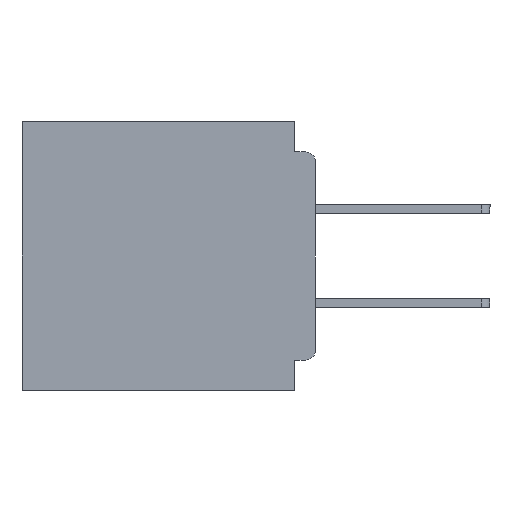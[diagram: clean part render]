
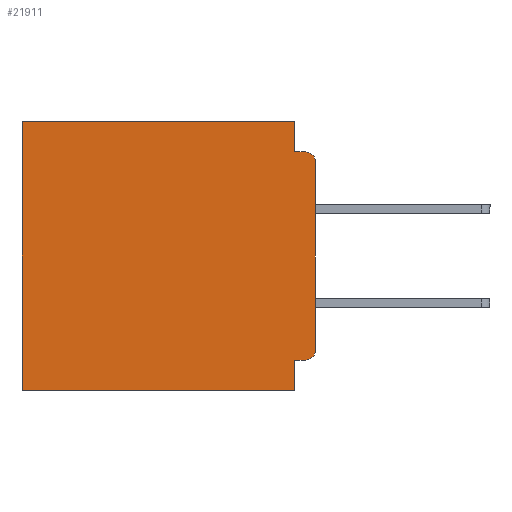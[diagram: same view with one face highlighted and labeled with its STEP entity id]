
A CAD part, left-side view. The second image highlights one B-rep face of the part: STEP entity #21911.
In plain terms, the highlighted planar face has unit normal (-1, 0, 0).
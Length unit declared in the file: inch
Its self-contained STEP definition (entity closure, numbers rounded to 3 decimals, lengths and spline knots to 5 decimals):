
#25 = EDGE_CURVE ( 'NONE', #33860, #26058, #36874, .T. ) ;
#89 = VERTEX_POINT ( 'NONE', #27693 ) ;
#97 = CARTESIAN_POINT ( 'NONE',  ( 0.3, 0.015, -0.06 ) ) ;
#1102 = VECTOR ( 'NONE', #43353, 39.37008 ) ;
#1605 = EDGE_CURVE ( 'NONE', #33860, #23498, #42872, .T. ) ;
#1631 = DIRECTION ( 'NONE',  ( 0., 0., -1. ) ) ;
#1905 = EDGE_CURVE ( 'NONE', #11350, #89, #7757, .T. ) ;
#2733 = ORIENTED_EDGE ( 'NONE', *, *, #29844, .F. ) ;
#2959 = DIRECTION ( 'NONE',  ( -1., 0., 0. ) ) ;
#3622 = CARTESIAN_POINT ( 'NONE',  ( 0.3, 0., -0.34 ) ) ;
#4730 = VECTOR ( 'NONE', #41948, 39.37008 ) ;
#5272 = CARTESIAN_POINT ( 'NONE',  ( 0.3, 0., -0.06 ) ) ;
#5467 = CARTESIAN_POINT ( 'NONE',  ( 0.3, 0.031, 0. ) ) ;
#6427 = AXIS2_PLACEMENT_3D ( 'NONE', #97, #45173, #18977 ) ;
#6617 = CARTESIAN_POINT ( 'NONE',  ( 0.3, 0.031, -0.4 ) ) ;
#6880 = ORIENTED_EDGE ( 'NONE', *, *, #1605, .F. ) ;
#7757 = LINE ( 'NONE', #12487, #46294 ) ;
#8088 = DIRECTION ( 'NONE',  ( 0., -1., 0. ) ) ;
#8098 = CARTESIAN_POINT ( 'NONE',  ( 0.3, 0.437, -0.4 ) ) ;
#9682 = CIRCLE ( 'NONE', #31097, 0.015 ) ;
#10049 = VERTEX_POINT ( 'NONE', #12297 ) ;
#11350 = VERTEX_POINT ( 'NONE', #5467 ) ;
#11752 = EDGE_LOOP ( 'NONE', ( #6880, #23285, #32112, #19750, #48287, #26219, #25047, #2733, #31502, #19133 ) ) ;
#11902 = VECTOR ( 'NONE', #24379, 39.37008 ) ;
#12297 = CARTESIAN_POINT ( 'NONE',  ( 0.3, 0.031, -0.045 ) ) ;
#12487 = CARTESIAN_POINT ( 'NONE',  ( 0.3, 0., 0. ) ) ;
#13491 = CARTESIAN_POINT ( 'NONE',  ( 0.3, 0.031, 0. ) ) ;
#15126 = EDGE_CURVE ( 'NONE', #20086, #39308, #40803, .T. ) ;
#15855 = CARTESIAN_POINT ( 'NONE',  ( 0.3, 0., -0.4 ) ) ;
#16086 = CARTESIAN_POINT ( 'NONE',  ( 0.3, 0.015, -0.355 ) ) ;
#16236 = DIRECTION ( 'NONE',  ( 1., 0., 0. ) ) ;
#16311 = VECTOR ( 'NONE', #46854, 39.37008 ) ;
#18798 = FACE_OUTER_BOUND ( 'NONE', #11752, .T. ) ;
#18823 = EDGE_CURVE ( 'NONE', #45656, #32060, #23514, .T. ) ;
#18977 = DIRECTION ( 'NONE',  ( 0., 0., -1. ) ) ;
#19133 = ORIENTED_EDGE ( 'NONE', *, *, #31142, .T. ) ;
#19750 = ORIENTED_EDGE ( 'NONE', *, *, #32361, .F. ) ;
#19763 = VECTOR ( 'NONE', #8088, 39.37008 ) ;
#19773 = VECTOR ( 'NONE', #24491, 39.37008 ) ;
#20086 = VERTEX_POINT ( 'NONE', #16086 ) ;
#20930 = LINE ( 'NONE', #30579, #19763 ) ;
#21177 = CARTESIAN_POINT ( 'NONE',  ( 0.3, 0., -0.4 ) ) ;
#21380 = AXIS2_PLACEMENT_3D ( 'NONE', #38627, #16236, #42326 ) ;
#21911 = ADVANCED_FACE ( 'NONE', ( #18798 ), #34909, .F. ) ;
#22479 = LINE ( 'NONE', #35400, #42313 ) ;
#23285 = ORIENTED_EDGE ( 'NONE', *, *, #25, .T. ) ;
#23498 = VERTEX_POINT ( 'NONE', #3622 ) ;
#23514 = LINE ( 'NONE', #15855, #4730 ) ;
#24379 = DIRECTION ( 'NONE',  ( 0., 0., -1. ) ) ;
#24491 = DIRECTION ( 'NONE',  ( 0., 1., 0. ) ) ;
#25047 = ORIENTED_EDGE ( 'NONE', *, *, #18823, .F. ) ;
#25414 = CARTESIAN_POINT ( 'NONE',  ( 0.3, 0.015, -0.34 ) ) ;
#25978 = EDGE_CURVE ( 'NONE', #89, #32060, #22479, .T. ) ;
#26058 = VERTEX_POINT ( 'NONE', #36025 ) ;
#26219 = ORIENTED_EDGE ( 'NONE', *, *, #25978, .T. ) ;
#27693 = CARTESIAN_POINT ( 'NONE',  ( 0.3, 0.437, 0. ) ) ;
#28641 = LINE ( 'NONE', #35745, #16311 ) ;
#29188 = DIRECTION ( 'NONE',  ( 0., 0., -1. ) ) ;
#29844 = EDGE_CURVE ( 'NONE', #39308, #45656, #28641, .T. ) ;
#30205 = EDGE_CURVE ( 'NONE', #10049, #26058, #20930, .T. ) ;
#30579 = CARTESIAN_POINT ( 'NONE',  ( 0.3, 0., -0.045 ) ) ;
#31097 = AXIS2_PLACEMENT_3D ( 'NONE', #25414, #2959, #29188 ) ;
#31142 = EDGE_CURVE ( 'NONE', #20086, #23498, #9682, .T. ) ;
#31502 = ORIENTED_EDGE ( 'NONE', *, *, #15126, .F. ) ;
#32060 = VERTEX_POINT ( 'NONE', #8098 ) ;
#32112 = ORIENTED_EDGE ( 'NONE', *, *, #30205, .F. ) ;
#32361 = EDGE_CURVE ( 'NONE', #11350, #10049, #40897, .T. ) ;
#33860 = VERTEX_POINT ( 'NONE', #5272 ) ;
#34909 = PLANE ( 'NONE',  #21380 ) ;
#35122 = DIRECTION ( 'NONE',  ( 0., 1., 0. ) ) ;
#35400 = CARTESIAN_POINT ( 'NONE',  ( 0.3, 0.437, -0.4 ) ) ;
#35745 = CARTESIAN_POINT ( 'NONE',  ( 0.3, 0.031, -0.4 ) ) ;
#36025 = CARTESIAN_POINT ( 'NONE',  ( 0.3, 0.015, -0.045 ) ) ;
#36874 = CIRCLE ( 'NONE', #6427, 0.015 ) ;
#38627 = CARTESIAN_POINT ( 'NONE',  ( 0.3, 0., -0.4 ) ) ;
#39308 = VERTEX_POINT ( 'NONE', #43916 ) ;
#40803 = LINE ( 'NONE', #43036, #19773 ) ;
#40897 = LINE ( 'NONE', #13491, #1102 ) ;
#41948 = DIRECTION ( 'NONE',  ( 0., 1., 0. ) ) ;
#42313 = VECTOR ( 'NONE', #1631, 39.37008 ) ;
#42326 = DIRECTION ( 'NONE',  ( 0., 0., -1. ) ) ;
#42872 = LINE ( 'NONE', #21177, #11902 ) ;
#43036 = CARTESIAN_POINT ( 'NONE',  ( 0.3, 0., -0.355 ) ) ;
#43353 = DIRECTION ( 'NONE',  ( 0., 0., -1. ) ) ;
#43916 = CARTESIAN_POINT ( 'NONE',  ( 0.3, 0.031, -0.355 ) ) ;
#45173 = DIRECTION ( 'NONE',  ( -1., 0., 0. ) ) ;
#45656 = VERTEX_POINT ( 'NONE', #6617 ) ;
#46294 = VECTOR ( 'NONE', #35122, 39.37008 ) ;
#46854 = DIRECTION ( 'NONE',  ( 0., 0., -1. ) ) ;
#48287 = ORIENTED_EDGE ( 'NONE', *, *, #1905, .T. ) ;
